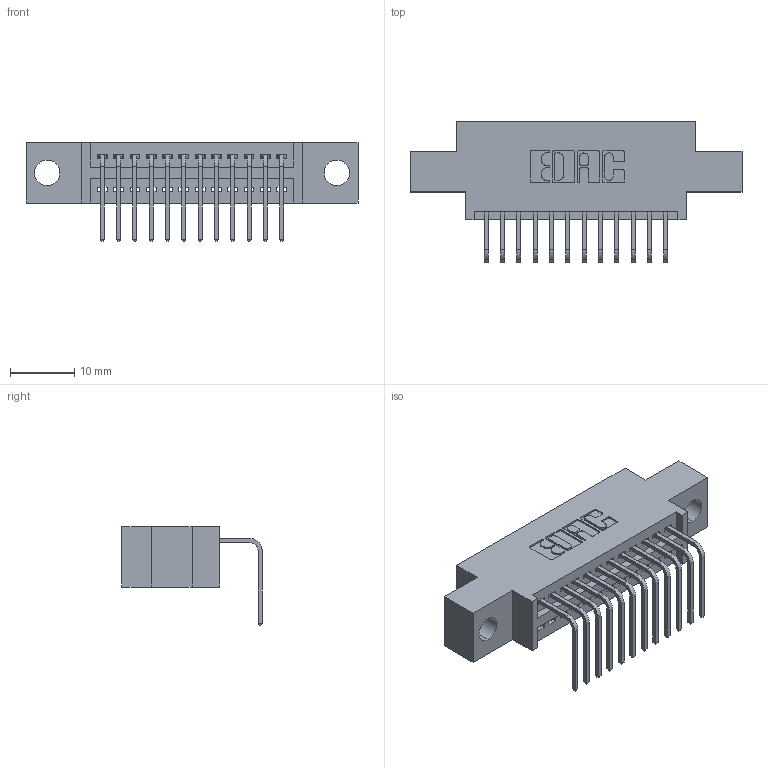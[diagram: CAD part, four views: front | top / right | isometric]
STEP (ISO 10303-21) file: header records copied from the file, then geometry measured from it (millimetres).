
FILE_DESCRIPTION (( 'STEP AP203' ), '1' );
FILE_NAME ('345-012-558-604.STEP', '2021-06-01T16:15:12', ( '' ), ( '' ), 'SwSTEP 2.0', 'SolidWorks 2020', '' );
FILE_SCHEMA (( 'CONFIG_CONTROL_DESIGN' ));
Length unit declared in the file: inch
Products named in the file (3): 345 Part_0.170 Offset - 0.156 Dia-TI; 345-292-001_558 Tail - 2; 345-012-558-604
Assembly tree (13 placements, depth 2):
  345-012-558-604
    345 Part_0.170 Offset - 0.156 Dia-TI
    345-292-001_558 Tail - 2  x12
Bounding box: 51.69 x 21.83 x 15.37 mm (x, y, z)
Volume: 4484.4 mm3; surface area: 5755.6 mm2
Topology: 13 solids, 13 shells, 864 faces, 2573 edges, 1698 vertices
Faces by surface type: plane 602, cylinder 262
Entity records: 13705 total; most frequent: CARTESIAN_POINT 2386, ORIENTED_EDGE 2330, DIRECTION 2125, EDGE_CURVE 1165, LINE 985, VECTOR 985, VERTEX_POINT 774, AXIS2_PLACEMENT_3D 570
